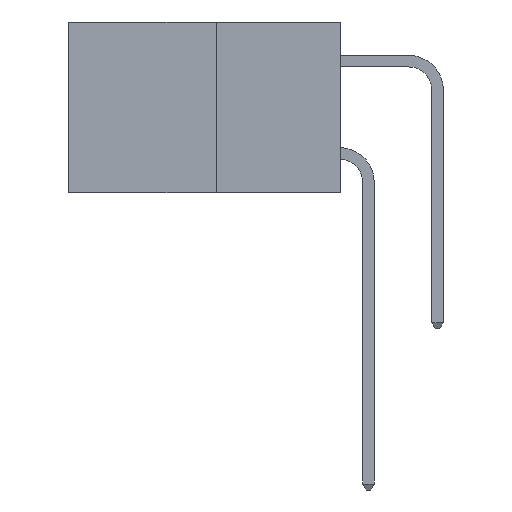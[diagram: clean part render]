
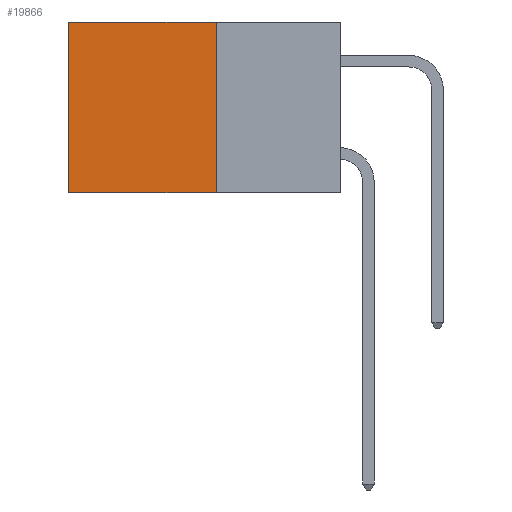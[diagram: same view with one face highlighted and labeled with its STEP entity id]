
A CAD part, left-side view. The second image highlights one B-rep face of the part: STEP entity #19866.
In plain terms, the highlighted planar face has unit normal (-1, 0, 0).
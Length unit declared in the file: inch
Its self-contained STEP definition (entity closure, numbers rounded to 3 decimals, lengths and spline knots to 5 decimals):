
#88 = CARTESIAN_POINT ( 'NONE',  ( 0.277, 0.27, -0.37 ) ) ;
#1397 = LINE ( 'NONE', #10234, #7295 ) ;
#3568 = EDGE_LOOP ( 'NONE', ( #17089, #13710, #11999, #11616 ) ) ;
#4076 = LINE ( 'NONE', #17806, #24797 ) ;
#5179 = VERTEX_POINT ( 'NONE', #15809 ) ;
#5791 = EDGE_CURVE ( 'NONE', #5179, #25197, #1397, .T. ) ;
#6056 = DIRECTION ( 'NONE',  ( 1., 0., 0. ) ) ;
#6880 = CARTESIAN_POINT ( 'NONE',  ( 0.277, 0.27, -0.37 ) ) ;
#7295 = VECTOR ( 'NONE', #23800, 39.37008 ) ;
#8552 = VECTOR ( 'NONE', #23180, 39.37008 ) ;
#8870 = VECTOR ( 'NONE', #24363, 39.37008 ) ;
#9491 = LINE ( 'NONE', #6880, #8870 ) ;
#9673 = EDGE_CURVE ( 'NONE', #5179, #11843, #9491, .T. ) ;
#9917 = EDGE_CURVE ( 'NONE', #25197, #22421, #18944, .T. ) ;
#10234 = CARTESIAN_POINT ( 'NONE',  ( 0.277, 0.27, 0. ) ) ;
#11064 = AXIS2_PLACEMENT_3D ( 'NONE', #88, #6056, #19723 ) ;
#11616 = ORIENTED_EDGE ( 'NONE', *, *, #5791, .T. ) ;
#11843 = VERTEX_POINT ( 'NONE', #22288 ) ;
#11999 = ORIENTED_EDGE ( 'NONE', *, *, #9673, .F. ) ;
#13710 = ORIENTED_EDGE ( 'NONE', *, *, #16766, .F. ) ;
#15401 = CARTESIAN_POINT ( 'NONE',  ( 0.277, 0.59, -0.37 ) ) ;
#15809 = CARTESIAN_POINT ( 'NONE',  ( 0.277, 0.27, 0. ) ) ;
#16766 = EDGE_CURVE ( 'NONE', #11843, #22421, #4076, .T. ) ;
#17089 = ORIENTED_EDGE ( 'NONE', *, *, #9917, .T. ) ;
#17391 = CARTESIAN_POINT ( 'NONE',  ( 0.277, 0.59, 0. ) ) ;
#17806 = CARTESIAN_POINT ( 'NONE',  ( 0.277, 0.27, -0.37 ) ) ;
#18806 = FACE_OUTER_BOUND ( 'NONE', #3568, .T. ) ;
#18944 = LINE ( 'NONE', #15401, #8552 ) ;
#19556 = PLANE ( 'NONE',  #11064 ) ;
#19723 = DIRECTION ( 'NONE',  ( 0., 0., -1. ) ) ;
#19760 = DIRECTION ( 'NONE',  ( 0., 1., 0. ) ) ;
#19866 = ADVANCED_FACE ( 'NONE', ( #18806 ), #19556, .F. ) ;
#22288 = CARTESIAN_POINT ( 'NONE',  ( 0.277, 0.27, -0.37 ) ) ;
#22421 = VERTEX_POINT ( 'NONE', #22731 ) ;
#22731 = CARTESIAN_POINT ( 'NONE',  ( 0.277, 0.59, -0.37 ) ) ;
#23180 = DIRECTION ( 'NONE',  ( 0., 0., -1. ) ) ;
#23800 = DIRECTION ( 'NONE',  ( 0., 1., 0. ) ) ;
#24363 = DIRECTION ( 'NONE',  ( 0., 0., -1. ) ) ;
#24797 = VECTOR ( 'NONE', #19760, 39.37008 ) ;
#25197 = VERTEX_POINT ( 'NONE', #17391 ) ;
